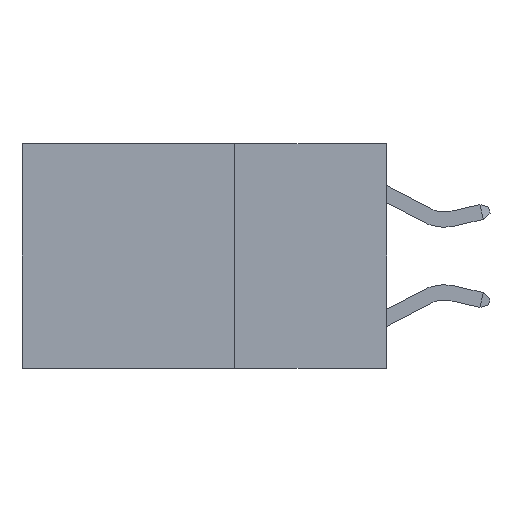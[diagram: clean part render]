
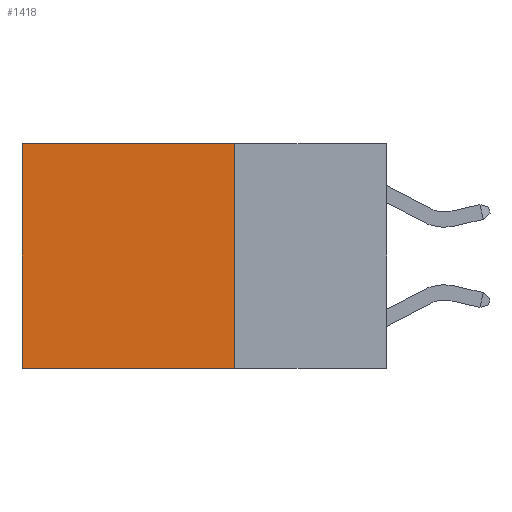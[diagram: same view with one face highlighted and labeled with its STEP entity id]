
A CAD part, left-side view. The second image highlights one B-rep face of the part: STEP entity #1418.
In plain terms, the highlighted planar face has unit normal (-1, 0, 0).
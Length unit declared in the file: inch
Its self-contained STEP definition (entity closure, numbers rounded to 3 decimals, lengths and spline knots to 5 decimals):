
#235 = VECTOR ( 'NONE', #1163, 39.37008 ) ;
#1163 = DIRECTION ( 'NONE',  ( 0., 0., -1. ) ) ;
#1418 = ADVANCED_FACE ( 'NONE', ( #2840 ), #11508, .F. ) ;
#1687 = ORIENTED_EDGE ( 'NONE', *, *, #12341, .T. ) ;
#1891 = VERTEX_POINT ( 'NONE', #6001 ) ;
#2063 = VERTEX_POINT ( 'NONE', #3663 ) ;
#2579 = LINE ( 'NONE', #3179, #12808 ) ;
#2840 = FACE_OUTER_BOUND ( 'NONE', #6370, .T. ) ;
#3137 = CARTESIAN_POINT ( 'NONE',  ( 0.2625, 0.25, -0.37 ) ) ;
#3179 = CARTESIAN_POINT ( 'NONE',  ( 0.2625, 0.6, 0. ) ) ;
#3663 = CARTESIAN_POINT ( 'NONE',  ( 0.2625, 0.6, 0. ) ) ;
#4635 = CARTESIAN_POINT ( 'NONE',  ( 0.2625, 0.25, -0.37 ) ) ;
#4954 = VECTOR ( 'NONE', #5623, 39.37008 ) ;
#5543 = VERTEX_POINT ( 'NONE', #11837 ) ;
#5623 = DIRECTION ( 'NONE',  ( 0., 1., 0. ) ) ;
#5882 = LINE ( 'NONE', #9406, #235 ) ;
#6001 = CARTESIAN_POINT ( 'NONE',  ( 0.2625, 0.6, -0.37 ) ) ;
#6210 = DIRECTION ( 'NONE',  ( 0., 0., -1. ) ) ;
#6370 = EDGE_LOOP ( 'NONE', ( #1687, #11282, #8082, #12040 ) ) ;
#6980 = EDGE_CURVE ( 'NONE', #5543, #12276, #5882, .T. ) ;
#7427 = CARTESIAN_POINT ( 'NONE',  ( 0.2625, 0.25, 0. ) ) ;
#7694 = EDGE_CURVE ( 'NONE', #12276, #1891, #12760, .T. ) ;
#8082 = ORIENTED_EDGE ( 'NONE', *, *, #6980, .F. ) ;
#8419 = DIRECTION ( 'NONE',  ( 0., 1., 0. ) ) ;
#8692 = AXIS2_PLACEMENT_3D ( 'NONE', #12188, #8881, #11454 ) ;
#8881 = DIRECTION ( 'NONE',  ( 1., 0., 0. ) ) ;
#9406 = CARTESIAN_POINT ( 'NONE',  ( 0.2625, 0.25, 0. ) ) ;
#11243 = VECTOR ( 'NONE', #8419, 39.37008 ) ;
#11282 = ORIENTED_EDGE ( 'NONE', *, *, #7694, .F. ) ;
#11454 = DIRECTION ( 'NONE',  ( 0., 0., -1. ) ) ;
#11508 = PLANE ( 'NONE',  #8692 ) ;
#11771 = EDGE_CURVE ( 'NONE', #5543, #2063, #13146, .T. ) ;
#11837 = CARTESIAN_POINT ( 'NONE',  ( 0.2625, 0.25, 0. ) ) ;
#12040 = ORIENTED_EDGE ( 'NONE', *, *, #11771, .T. ) ;
#12188 = CARTESIAN_POINT ( 'NONE',  ( 0.2625, 0.25, 0. ) ) ;
#12276 = VERTEX_POINT ( 'NONE', #3137 ) ;
#12341 = EDGE_CURVE ( 'NONE', #2063, #1891, #2579, .T. ) ;
#12760 = LINE ( 'NONE', #4635, #4954 ) ;
#12808 = VECTOR ( 'NONE', #6210, 39.37008 ) ;
#13146 = LINE ( 'NONE', #7427, #11243 ) ;
